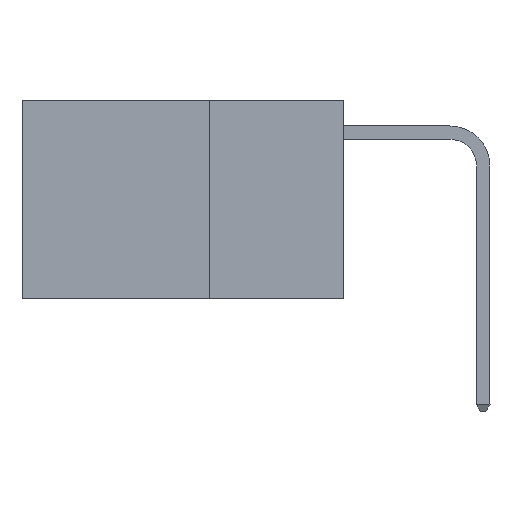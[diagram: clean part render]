
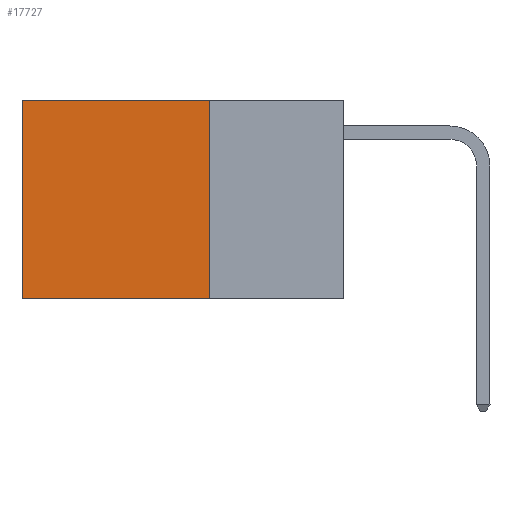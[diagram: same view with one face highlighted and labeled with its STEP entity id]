
A CAD part, left-side view. The second image highlights one B-rep face of the part: STEP entity #17727.
In plain terms, the highlighted planar face has unit normal (-1, 0, 0).
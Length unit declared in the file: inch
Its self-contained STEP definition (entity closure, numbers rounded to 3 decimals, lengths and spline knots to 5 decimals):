
#95 = EDGE_LOOP ( 'NONE', ( #6394, #10009, #15714, #10862 ) ) ;
#661 = CARTESIAN_POINT ( 'NONE',  ( 0.2625, 0.6, 0. ) ) ;
#1979 = LINE ( 'NONE', #10893, #7719 ) ;
#2033 = DIRECTION ( 'NONE',  ( 0., 1., 0. ) ) ;
#2864 = PLANE ( 'NONE',  #8986 ) ;
#4613 = DIRECTION ( 'NONE',  ( 1., 0., 0. ) ) ;
#4653 = DIRECTION ( 'NONE',  ( 0., 0., -1. ) ) ;
#4812 = CARTESIAN_POINT ( 'NONE',  ( 0.2625, 0.25, -0.37 ) ) ;
#5168 = CARTESIAN_POINT ( 'NONE',  ( 0.2625, 0.25, -0.37 ) ) ;
#5448 = EDGE_CURVE ( 'NONE', #8726, #12233, #18532, .T. ) ;
#5525 = VERTEX_POINT ( 'NONE', #17575 ) ;
#6394 = ORIENTED_EDGE ( 'NONE', *, *, #5448, .T. ) ;
#6693 = EDGE_CURVE ( 'NONE', #5525, #7147, #1979, .T. ) ;
#7147 = VERTEX_POINT ( 'NONE', #4812 ) ;
#7380 = DIRECTION ( 'NONE',  ( 0., 1., 0. ) ) ;
#7719 = VECTOR ( 'NONE', #4653, 39.37008 ) ;
#7768 = VECTOR ( 'NONE', #2033, 39.37008 ) ;
#8726 = VERTEX_POINT ( 'NONE', #14662 ) ;
#8986 = AXIS2_PLACEMENT_3D ( 'NONE', #11858, #4613, #17805 ) ;
#9571 = LINE ( 'NONE', #5168, #7768 ) ;
#10009 = ORIENTED_EDGE ( 'NONE', *, *, #12436, .F. ) ;
#10862 = ORIENTED_EDGE ( 'NONE', *, *, #15690, .T. ) ;
#10893 = CARTESIAN_POINT ( 'NONE',  ( 0.2625, 0.25, 0. ) ) ;
#11120 = DIRECTION ( 'NONE',  ( 0., 0., -1. ) ) ;
#11478 = CARTESIAN_POINT ( 'NONE',  ( 0.2625, 0.6, -0.37 ) ) ;
#11797 = LINE ( 'NONE', #17753, #19211 ) ;
#11858 = CARTESIAN_POINT ( 'NONE',  ( 0.2625, 0.25, 0. ) ) ;
#12233 = VERTEX_POINT ( 'NONE', #11478 ) ;
#12436 = EDGE_CURVE ( 'NONE', #7147, #12233, #9571, .T. ) ;
#13895 = VECTOR ( 'NONE', #11120, 39.37008 ) ;
#14662 = CARTESIAN_POINT ( 'NONE',  ( 0.2625, 0.6, 0. ) ) ;
#15690 = EDGE_CURVE ( 'NONE', #5525, #8726, #11797, .T. ) ;
#15714 = ORIENTED_EDGE ( 'NONE', *, *, #6693, .F. ) ;
#17575 = CARTESIAN_POINT ( 'NONE',  ( 0.2625, 0.25, 0. ) ) ;
#17727 = ADVANCED_FACE ( 'NONE', ( #17988 ), #2864, .F. ) ;
#17753 = CARTESIAN_POINT ( 'NONE',  ( 0.2625, 0.25, 0. ) ) ;
#17805 = DIRECTION ( 'NONE',  ( 0., 0., -1. ) ) ;
#17988 = FACE_OUTER_BOUND ( 'NONE', #95, .T. ) ;
#18532 = LINE ( 'NONE', #661, #13895 ) ;
#19211 = VECTOR ( 'NONE', #7380, 39.37008 ) ;
